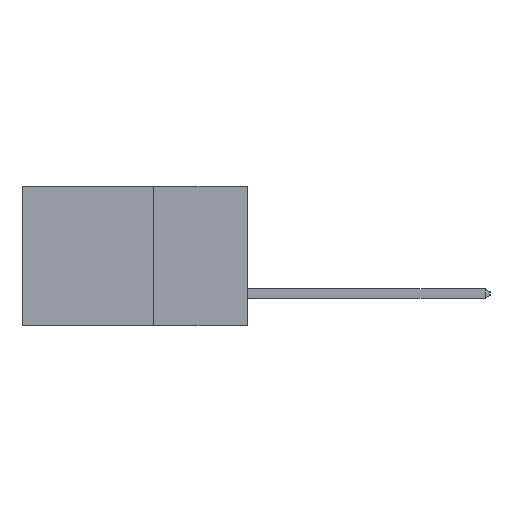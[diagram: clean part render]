
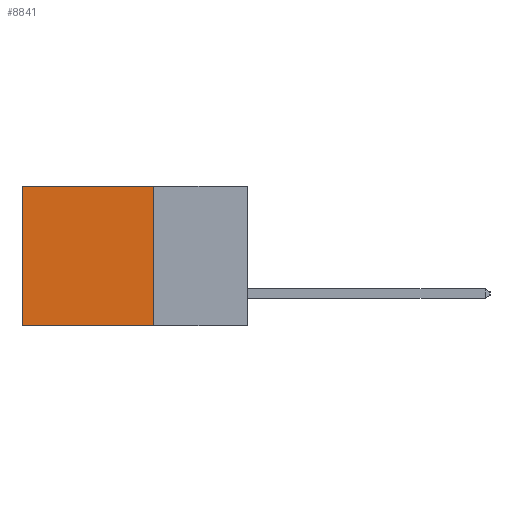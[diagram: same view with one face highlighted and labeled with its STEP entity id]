
A CAD part, left-side view. The second image highlights one B-rep face of the part: STEP entity #8841.
In plain terms, the highlighted planar face has unit normal (-1, 0, 0).
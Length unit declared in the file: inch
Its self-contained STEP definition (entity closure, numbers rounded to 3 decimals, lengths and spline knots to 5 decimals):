
#360 = CARTESIAN_POINT ( 'NONE',  ( 0.2615, 0.6, -0.37 ) ) ;
#365 = VERTEX_POINT ( 'NONE', #8121 ) ;
#1196 = DIRECTION ( 'NONE',  ( 0., 0., -1. ) ) ;
#1919 = VECTOR ( 'NONE', #4515, 39.37008 ) ;
#2231 = ORIENTED_EDGE ( 'NONE', *, *, #2381, .F. ) ;
#2349 = LINE ( 'NONE', #3134, #11363 ) ;
#2370 = DIRECTION ( 'NONE',  ( 0., 0., -1. ) ) ;
#2375 = VECTOR ( 'NONE', #2370, 39.37008 ) ;
#2381 = EDGE_CURVE ( 'NONE', #365, #6207, #2416, .T. ) ;
#2416 = LINE ( 'NONE', #10296, #9193 ) ;
#2451 = CARTESIAN_POINT ( 'NONE',  ( 0.2615, 0.25, -0.37 ) ) ;
#2690 = AXIS2_PLACEMENT_3D ( 'NONE', #7457, #6621, #1196 ) ;
#2824 = CARTESIAN_POINT ( 'NONE',  ( 0.2615, 0.25, 0. ) ) ;
#3134 = CARTESIAN_POINT ( 'NONE',  ( 0.2615, 0.6, -0.37 ) ) ;
#3186 = FACE_OUTER_BOUND ( 'NONE', #6319, .T. ) ;
#3274 = ORIENTED_EDGE ( 'NONE', *, *, #4813, .F. ) ;
#3292 = VERTEX_POINT ( 'NONE', #2824 ) ;
#3548 = ORIENTED_EDGE ( 'NONE', *, *, #8936, .T. ) ;
#4044 = LINE ( 'NONE', #9690, #1919 ) ;
#4147 = ORIENTED_EDGE ( 'NONE', *, *, #9225, .T. ) ;
#4515 = DIRECTION ( 'NONE',  ( 0., 1., 0. ) ) ;
#4810 = LINE ( 'NONE', #2451, #2375 ) ;
#4813 = EDGE_CURVE ( 'NONE', #3292, #365, #4810, .T. ) ;
#5740 = PLANE ( 'NONE',  #2690 ) ;
#6207 = VERTEX_POINT ( 'NONE', #360 ) ;
#6319 = EDGE_LOOP ( 'NONE', ( #3548, #2231, #3274, #4147 ) ) ;
#6621 = DIRECTION ( 'NONE',  ( 1., 0., 0. ) ) ;
#6804 = CARTESIAN_POINT ( 'NONE',  ( 0.2615, 0.6, 0. ) ) ;
#6991 = DIRECTION ( 'NONE',  ( 0., 1., 0. ) ) ;
#7457 = CARTESIAN_POINT ( 'NONE',  ( 0.2615, 0.25, -0.37 ) ) ;
#8121 = CARTESIAN_POINT ( 'NONE',  ( 0.2615, 0.25, -0.37 ) ) ;
#8444 = DIRECTION ( 'NONE',  ( 0., 0., -1. ) ) ;
#8841 = ADVANCED_FACE ( 'NONE', ( #3186 ), #5740, .F. ) ;
#8936 = EDGE_CURVE ( 'NONE', #9604, #6207, #2349, .T. ) ;
#9193 = VECTOR ( 'NONE', #6991, 39.37008 ) ;
#9225 = EDGE_CURVE ( 'NONE', #3292, #9604, #4044, .T. ) ;
#9604 = VERTEX_POINT ( 'NONE', #6804 ) ;
#9690 = CARTESIAN_POINT ( 'NONE',  ( 0.2615, 0.25, 0. ) ) ;
#10296 = CARTESIAN_POINT ( 'NONE',  ( 0.2615, 0.25, -0.37 ) ) ;
#11363 = VECTOR ( 'NONE', #8444, 39.37008 ) ;
